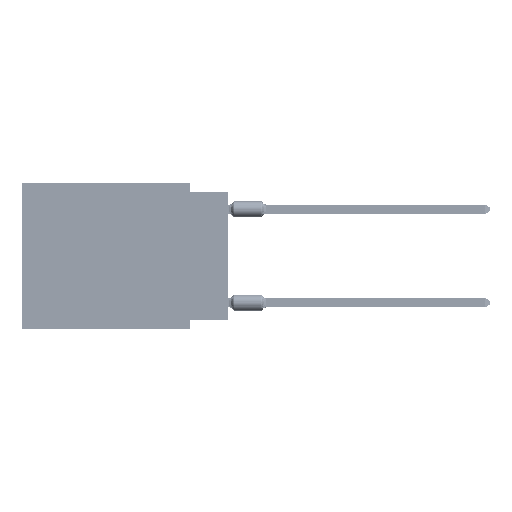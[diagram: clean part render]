
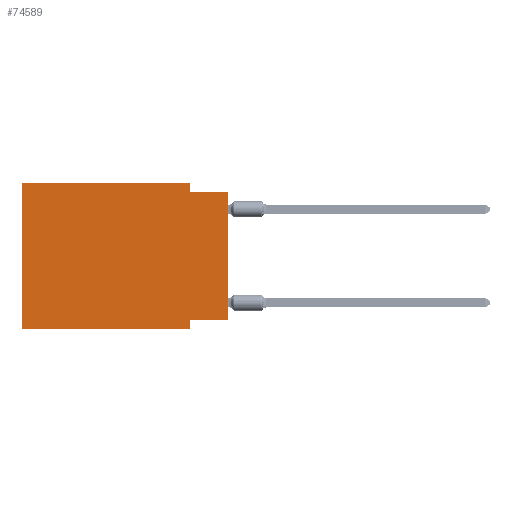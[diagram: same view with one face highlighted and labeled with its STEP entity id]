
A CAD part, left-side view. The second image highlights one B-rep face of the part: STEP entity #74589.
In plain terms, the highlighted planar face has unit normal (-1, 0, 0).
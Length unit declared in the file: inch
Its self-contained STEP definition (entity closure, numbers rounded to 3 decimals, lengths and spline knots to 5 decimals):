
#414 = VERTEX_POINT ( 'NONE', #77436 ) ;
#1469 = CARTESIAN_POINT ( 'NONE',  ( 0., 0., -0.025 ) ) ;
#2201 = ORIENTED_EDGE ( 'NONE', *, *, #24173, .T. ) ;
#4176 = DIRECTION ( 'NONE',  ( 0., 0., -1. ) ) ;
#5837 = EDGE_CURVE ( 'NONE', #414, #21151, #47576, .T. ) ;
#6214 = EDGE_LOOP ( 'NONE', ( #2201, #19180, #44485, #26544, #77133, #75182, #10502, #13726 ) ) ;
#7318 = LINE ( 'NONE', #71596, #41618 ) ;
#7846 = CARTESIAN_POINT ( 'NONE',  ( 0., 0.55, 0. ) ) ;
#8294 = DIRECTION ( 'NONE',  ( 1., 0., 0. ) ) ;
#8880 = LINE ( 'NONE', #74711, #35751 ) ;
#10502 = ORIENTED_EDGE ( 'NONE', *, *, #23844, .F. ) ;
#11383 = LINE ( 'NONE', #40391, #36917 ) ;
#13046 = DIRECTION ( 'NONE',  ( 0., 0., 1. ) ) ;
#13726 = ORIENTED_EDGE ( 'NONE', *, *, #70169, .F. ) ;
#14605 = VERTEX_POINT ( 'NONE', #17193 ) ;
#17193 = CARTESIAN_POINT ( 'NONE',  ( 0., 0.55, -0.39 ) ) ;
#18811 = DIRECTION ( 'NONE',  ( 0., -1., 0. ) ) ;
#19180 = ORIENTED_EDGE ( 'NONE', *, *, #42664, .F. ) ;
#19612 = EDGE_CURVE ( 'NONE', #14605, #26843, #7318, .T. ) ;
#21151 = VERTEX_POINT ( 'NONE', #70374 ) ;
#21753 = CARTESIAN_POINT ( 'NONE',  ( 0., 0., -0.365 ) ) ;
#23127 = DIRECTION ( 'NONE',  ( 0., 0., 1. ) ) ;
#23844 = EDGE_CURVE ( 'NONE', #74267, #26843, #58219, .T. ) ;
#24173 = EDGE_CURVE ( 'NONE', #29951, #24804, #11383, .T. ) ;
#24804 = VERTEX_POINT ( 'NONE', #1469 ) ;
#25540 = PLANE ( 'NONE',  #31685 ) ;
#26513 = VECTOR ( 'NONE', #4176, 39.37008 ) ;
#26544 = ORIENTED_EDGE ( 'NONE', *, *, #55015, .F. ) ;
#26843 = VERTEX_POINT ( 'NONE', #36918 ) ;
#29951 = VERTEX_POINT ( 'NONE', #21753 ) ;
#30879 = VECTOR ( 'NONE', #13046, 39.37008 ) ;
#31685 = AXIS2_PLACEMENT_3D ( 'NONE', #61995, #8294, #67089 ) ;
#31808 = VECTOR ( 'NONE', #40927, 39.37008 ) ;
#32129 = LINE ( 'NONE', #7846, #45161 ) ;
#35751 = VECTOR ( 'NONE', #68839, 39.37008 ) ;
#36917 = VECTOR ( 'NONE', #23127, 39.37008 ) ;
#36918 = CARTESIAN_POINT ( 'NONE',  ( 0., 0.1, -0.39 ) ) ;
#40391 = CARTESIAN_POINT ( 'NONE',  ( 0., 0., 0. ) ) ;
#40580 = CARTESIAN_POINT ( 'NONE',  ( 0., 0.1, -0.39 ) ) ;
#40927 = DIRECTION ( 'NONE',  ( 0., 0., -1. ) ) ;
#41618 = VECTOR ( 'NONE', #42204, 39.37008 ) ;
#42204 = DIRECTION ( 'NONE',  ( 0., -1., 0. ) ) ;
#42664 = EDGE_CURVE ( 'NONE', #21151, #24804, #57108, .T. ) ;
#44485 = ORIENTED_EDGE ( 'NONE', *, *, #5837, .F. ) ;
#45161 = VECTOR ( 'NONE', #18811, 39.37008 ) ;
#45166 = VERTEX_POINT ( 'NONE', #52849 ) ;
#47576 = LINE ( 'NONE', #76222, #31808 ) ;
#50854 = DIRECTION ( 'NONE',  ( 0., -1., 0. ) ) ;
#52849 = CARTESIAN_POINT ( 'NONE',  ( 0., 0.55, 0. ) ) ;
#55015 = EDGE_CURVE ( 'NONE', #45166, #414, #32129, .T. ) ;
#56730 = CARTESIAN_POINT ( 'NONE',  ( 0., 0., -0.025 ) ) ;
#57108 = LINE ( 'NONE', #56730, #58990 ) ;
#58219 = LINE ( 'NONE', #40580, #26513 ) ;
#58990 = VECTOR ( 'NONE', #50854, 39.37008 ) ;
#60856 = CARTESIAN_POINT ( 'NONE',  ( 0., 0.55, 0. ) ) ;
#61995 = CARTESIAN_POINT ( 'NONE',  ( 0., 0.55, 0. ) ) ;
#66729 = LINE ( 'NONE', #60856, #30879 ) ;
#67089 = DIRECTION ( 'NONE',  ( 0., 0., -1. ) ) ;
#68839 = DIRECTION ( 'NONE',  ( 0., 1., 0. ) ) ;
#70169 = EDGE_CURVE ( 'NONE', #29951, #74267, #8880, .T. ) ;
#70374 = CARTESIAN_POINT ( 'NONE',  ( 0., 0.1, -0.025 ) ) ;
#71596 = CARTESIAN_POINT ( 'NONE',  ( 0., 0.55, -0.39 ) ) ;
#72064 = EDGE_CURVE ( 'NONE', #14605, #45166, #66729, .T. ) ;
#74121 = FACE_OUTER_BOUND ( 'NONE', #6214, .T. ) ;
#74267 = VERTEX_POINT ( 'NONE', #75379 ) ;
#74589 = ADVANCED_FACE ( 'NONE', ( #74121 ), #25540, .F. ) ;
#74711 = CARTESIAN_POINT ( 'NONE',  ( 0., 0., -0.365 ) ) ;
#75182 = ORIENTED_EDGE ( 'NONE', *, *, #19612, .T. ) ;
#75379 = CARTESIAN_POINT ( 'NONE',  ( 0., 0.1, -0.365 ) ) ;
#76222 = CARTESIAN_POINT ( 'NONE',  ( 0., 0.1, 0. ) ) ;
#77133 = ORIENTED_EDGE ( 'NONE', *, *, #72064, .F. ) ;
#77436 = CARTESIAN_POINT ( 'NONE',  ( 0., 0.1, 0. ) ) ;
